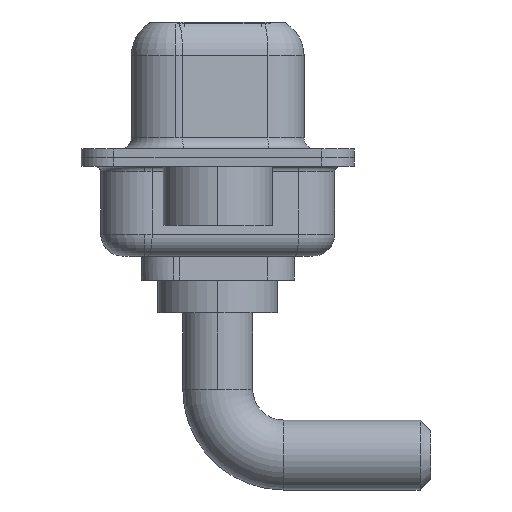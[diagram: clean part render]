
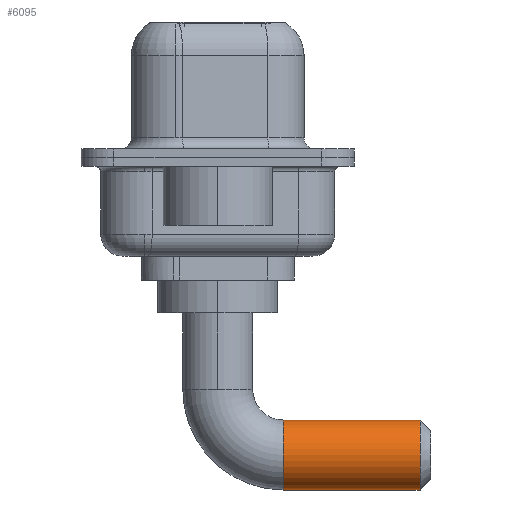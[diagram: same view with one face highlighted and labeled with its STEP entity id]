
A CAD part, left-side view. The second image highlights one B-rep face of the part: STEP entity #6095.
In plain terms, the highlighted cylindrical face has radius 1.6 mm (diameter 3.2 mm), a partial arc.
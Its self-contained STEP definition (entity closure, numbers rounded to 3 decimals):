
#94 = CARTESIAN_POINT ( 'NONE',  ( 0., -3., -4.9 ) ) ;
#243 = FACE_OUTER_BOUND ( 'NONE', #5513, .T. ) ;
#495 = EDGE_CURVE ( 'NONE', #7835, #5720, #4839, .T. ) ;
#501 = CARTESIAN_POINT ( 'NONE',  ( 0., -9.25, -4.9 ) ) ;
#1226 = AXIS2_PLACEMENT_3D ( 'NONE', #7907, #8682, #12017 ) ;
#1398 = ORIENTED_EDGE ( 'NONE', *, *, #495, .F. ) ;
#1643 = VECTOR ( 'NONE', #3813, 1000. ) ;
#1958 = ORIENTED_EDGE ( 'NONE', *, *, #9968, .T. ) ;
#2257 = CIRCLE ( 'NONE', #1226, 1.6 ) ;
#3046 = DIRECTION ( 'NONE',  ( -1., 0., 0. ) ) ;
#3269 = ORIENTED_EDGE ( 'NONE', *, *, #4081, .T. ) ;
#3662 = CIRCLE ( 'NONE', #6741, 1.6 ) ;
#3723 = VECTOR ( 'NONE', #12629, 1000. ) ;
#3813 = DIRECTION ( 'NONE',  ( 0., -1., 0. ) ) ;
#3889 = DIRECTION ( 'NONE',  ( 0., -1., 0. ) ) ;
#4081 = EDGE_CURVE ( 'NONE', #7835, #12620, #3662, .T. ) ;
#4335 = CYLINDRICAL_SURFACE ( 'NONE', #9027, 1.6 ) ;
#4839 = LINE ( 'NONE', #11745, #1643 ) ;
#5513 = EDGE_LOOP ( 'NONE', ( #1398, #3269, #1958, #9150 ) ) ;
#5720 = VERTEX_POINT ( 'NONE', #501 ) ;
#6095 = ADVANCED_FACE ( 'NONE', ( #243 ), #4335, .T. ) ;
#6741 = AXIS2_PLACEMENT_3D ( 'NONE', #7897, #3889, #3046 ) ;
#7239 = DIRECTION ( 'NONE',  ( 0., -1., 0. ) ) ;
#7835 = VERTEX_POINT ( 'NONE', #94 ) ;
#7864 = CARTESIAN_POINT ( 'NONE',  ( 0., -3., -8.1 ) ) ;
#7897 = CARTESIAN_POINT ( 'NONE',  ( 0., -3., -6.5 ) ) ;
#7907 = CARTESIAN_POINT ( 'NONE',  ( 0., -9.25, -6.5 ) ) ;
#8273 = DIRECTION ( 'NONE',  ( 0., 0., -1. ) ) ;
#8682 = DIRECTION ( 'NONE',  ( 0., 1., 0. ) ) ;
#8882 = LINE ( 'NONE', #7864, #3723 ) ;
#9027 = AXIS2_PLACEMENT_3D ( 'NONE', #10246, #7239, #8273 ) ;
#9150 = ORIENTED_EDGE ( 'NONE', *, *, #10438, .T. ) ;
#9842 = CARTESIAN_POINT ( 'NONE',  ( 0., -9.25, -8.1 ) ) ;
#9968 = EDGE_CURVE ( 'NONE', #12620, #10029, #8882, .T. ) ;
#10029 = VERTEX_POINT ( 'NONE', #9842 ) ;
#10246 = CARTESIAN_POINT ( 'NONE',  ( 0., -3., -6.5 ) ) ;
#10438 = EDGE_CURVE ( 'NONE', #10029, #5720, #2257, .T. ) ;
#11745 = CARTESIAN_POINT ( 'NONE',  ( 0., -3., -4.9 ) ) ;
#12017 = DIRECTION ( 'NONE',  ( 0., 0., -1. ) ) ;
#12209 = CARTESIAN_POINT ( 'NONE',  ( 0., -3., -8.1 ) ) ;
#12620 = VERTEX_POINT ( 'NONE', #12209 ) ;
#12629 = DIRECTION ( 'NONE',  ( 0., -1., 0. ) ) ;
